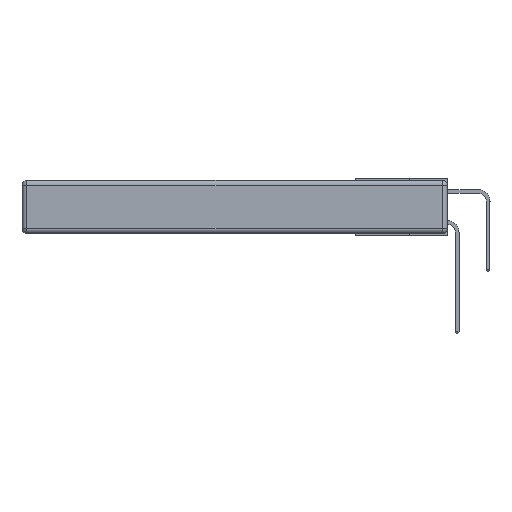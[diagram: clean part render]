
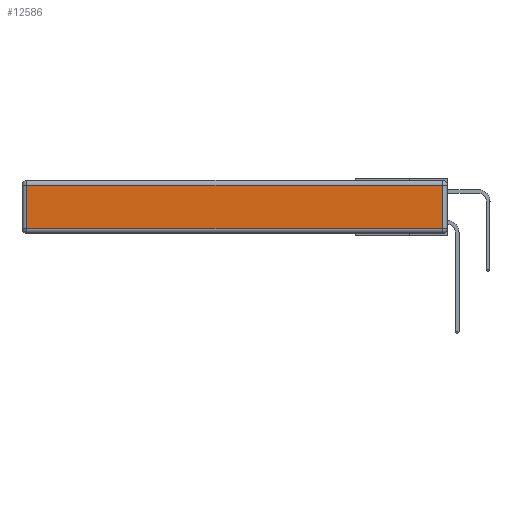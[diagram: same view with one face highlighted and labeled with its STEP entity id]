
A CAD part, left-side view. The second image highlights one B-rep face of the part: STEP entity #12586.
In plain terms, the highlighted planar face has unit normal (-1, 0, 0).
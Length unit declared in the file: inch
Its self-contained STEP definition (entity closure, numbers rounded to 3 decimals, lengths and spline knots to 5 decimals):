
#91 = EDGE_CURVE ( 'NONE', #857, #8468, #9058, .T. ) ;
#638 = CARTESIAN_POINT ( 'NONE',  ( 0., 2.72, -0.343 ) ) ;
#857 = VERTEX_POINT ( 'NONE', #9952 ) ;
#955 = DIRECTION ( 'NONE',  ( -1., 0., 0. ) ) ;
#2122 = EDGE_CURVE ( 'NONE', #10488, #11106, #5465, .T. ) ;
#2162 = EDGE_CURVE ( 'NONE', #11106, #857, #10496, .T. ) ;
#2575 = FACE_OUTER_BOUND ( 'NONE', #13012, .T. ) ;
#2577 = VECTOR ( 'NONE', #7742, 39.37008 ) ;
#2584 = CARTESIAN_POINT ( 'NONE',  ( 0., 2.72, -0.03 ) ) ;
#2603 = ORIENTED_EDGE ( 'NONE', *, *, #2162, .T. ) ;
#2605 = AXIS2_PLACEMENT_3D ( 'NONE', #7286, #955, #7344 ) ;
#2890 = EDGE_CURVE ( 'NONE', #8468, #10488, #8200, .T. ) ;
#3051 = ORIENTED_EDGE ( 'NONE', *, *, #2890, .T. ) ;
#3508 = DIRECTION ( 'NONE',  ( 0., 0., 1. ) ) ;
#5042 = CARTESIAN_POINT ( 'NONE',  ( 0., 2.72, -0.313 ) ) ;
#5465 = LINE ( 'NONE', #12969, #2577 ) ;
#6776 = CARTESIAN_POINT ( 'NONE',  ( 0., 0.03, -0.313 ) ) ;
#6791 = CARTESIAN_POINT ( 'NONE',  ( 0., 0.03, -0.343 ) ) ;
#7286 = CARTESIAN_POINT ( 'NONE',  ( 0., 0., -0.343 ) ) ;
#7344 = DIRECTION ( 'NONE',  ( 0., 0., 1. ) ) ;
#7712 = VECTOR ( 'NONE', #12643, 39.37008 ) ;
#7742 = DIRECTION ( 'NONE',  ( 0., -1., 0. ) ) ;
#8152 = VECTOR ( 'NONE', #3508, 39.37008 ) ;
#8200 = LINE ( 'NONE', #638, #7712 ) ;
#8242 = ORIENTED_EDGE ( 'NONE', *, *, #2122, .T. ) ;
#8468 = VERTEX_POINT ( 'NONE', #2584 ) ;
#9058 = LINE ( 'NONE', #10059, #13658 ) ;
#9425 = PLANE ( 'NONE',  #2605 ) ;
#9952 = CARTESIAN_POINT ( 'NONE',  ( 0., 0.03, -0.03 ) ) ;
#10059 = CARTESIAN_POINT ( 'NONE',  ( 0., 2.75, -0.03 ) ) ;
#10488 = VERTEX_POINT ( 'NONE', #5042 ) ;
#10496 = LINE ( 'NONE', #6791, #8152 ) ;
#11025 = DIRECTION ( 'NONE',  ( 0., 1., 0. ) ) ;
#11106 = VERTEX_POINT ( 'NONE', #6776 ) ;
#12422 = ORIENTED_EDGE ( 'NONE', *, *, #91, .T. ) ;
#12586 = ADVANCED_FACE ( 'NONE', ( #2575 ), #9425, .T. ) ;
#12643 = DIRECTION ( 'NONE',  ( 0., 0., -1. ) ) ;
#12969 = CARTESIAN_POINT ( 'NONE',  ( 0., 0., -0.313 ) ) ;
#13012 = EDGE_LOOP ( 'NONE', ( #8242, #2603, #12422, #3051 ) ) ;
#13658 = VECTOR ( 'NONE', #11025, 39.37008 ) ;
